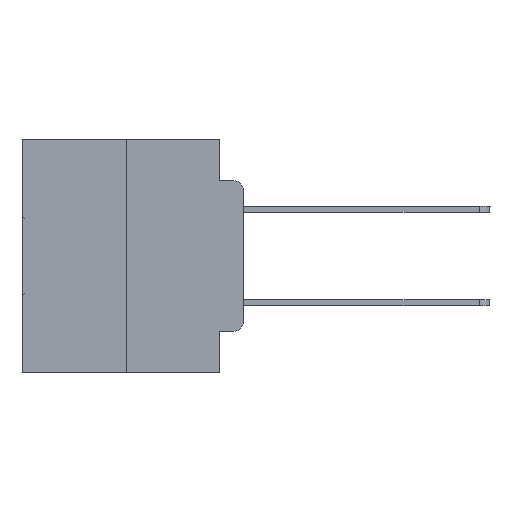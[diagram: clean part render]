
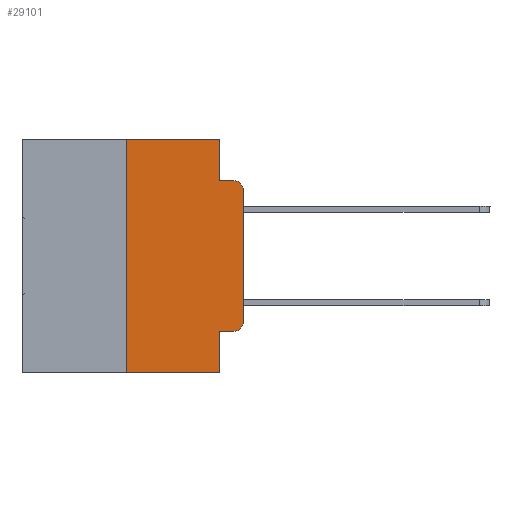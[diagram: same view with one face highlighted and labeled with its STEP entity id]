
A CAD part, left-side view. The second image highlights one B-rep face of the part: STEP entity #29101.
In plain terms, the highlighted planar face has unit normal (-1, 0, 0).
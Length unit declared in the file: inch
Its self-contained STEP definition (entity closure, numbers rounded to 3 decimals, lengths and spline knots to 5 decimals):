
#523 = ORIENTED_EDGE ( 'NONE', *, *, #27543, .T. ) ;
#621 = VERTEX_POINT ( 'NONE', #14830 ) ;
#1143 = CARTESIAN_POINT ( 'NONE',  ( 0., 0.473, 0. ) ) ;
#1203 = VERTEX_POINT ( 'NONE', #7807 ) ;
#1286 = EDGE_LOOP ( 'NONE', ( #523, #7363, #1351, #14677, #22027, #17001, #29893, #12021, #25044, #13533 ) ) ;
#1342 = VERTEX_POINT ( 'NONE', #10955 ) ;
#1351 = ORIENTED_EDGE ( 'NONE', *, *, #3787, .F. ) ;
#1539 = EDGE_CURVE ( 'NONE', #4586, #14637, #24860, .T. ) ;
#1832 = VERTEX_POINT ( 'NONE', #7961 ) ;
#2256 = VECTOR ( 'NONE', #30206, 39.37008 ) ;
#2321 = LINE ( 'NONE', #16980, #14815 ) ;
#2412 = CIRCLE ( 'NONE', #7745, 0.02 ) ;
#2580 = VERTEX_POINT ( 'NONE', #20809 ) ;
#3767 = CARTESIAN_POINT ( 'NONE',  ( 0., 0.051, 0. ) ) ;
#3774 = DIRECTION ( 'NONE',  ( 0., -1., 0. ) ) ;
#3787 = EDGE_CURVE ( 'NONE', #8110, #12003, #15507, .T. ) ;
#3994 = DIRECTION ( 'NONE',  ( 0., -1., 0. ) ) ;
#4586 = VERTEX_POINT ( 'NONE', #30674 ) ;
#6032 = CARTESIAN_POINT ( 'NONE',  ( 0., 0.051, -0.5 ) ) ;
#6189 = LINE ( 'NONE', #25192, #30608 ) ;
#7363 = ORIENTED_EDGE ( 'NONE', *, *, #24331, .T. ) ;
#7745 = AXIS2_PLACEMENT_3D ( 'NONE', #24017, #9310, #26421 ) ;
#7807 = CARTESIAN_POINT ( 'NONE',  ( 0., 0., -0.3915 ) ) ;
#7961 = CARTESIAN_POINT ( 'NONE',  ( 0., 0.25, 0. ) ) ;
#8110 = VERTEX_POINT ( 'NONE', #28149 ) ;
#8748 = VECTOR ( 'NONE', #28116, 39.37008 ) ;
#8820 = DIRECTION ( 'NONE',  ( 1., 0., 0. ) ) ;
#9310 = DIRECTION ( 'NONE',  ( -1., 0., 0. ) ) ;
#9916 = CARTESIAN_POINT ( 'NONE',  ( 0., 0.02, -0.1085 ) ) ;
#10564 = AXIS2_PLACEMENT_3D ( 'NONE', #20979, #8820, #25940 ) ;
#10860 = CARTESIAN_POINT ( 'NONE',  ( 0., 0.051, -0.0885 ) ) ;
#10955 = CARTESIAN_POINT ( 'NONE',  ( 0., 0., -0.1085 ) ) ;
#11109 = EDGE_CURVE ( 'NONE', #4586, #1832, #2321, .T. ) ;
#11284 = VERTEX_POINT ( 'NONE', #19986 ) ;
#12003 = VERTEX_POINT ( 'NONE', #17802 ) ;
#12021 = ORIENTED_EDGE ( 'NONE', *, *, #31860, .F. ) ;
#12216 = CARTESIAN_POINT ( 'NONE',  ( 0., 0.051, -0.4115 ) ) ;
#12369 = DIRECTION ( 'NONE',  ( 0., 0., -1. ) ) ;
#12460 = LINE ( 'NONE', #3767, #25475 ) ;
#13533 = ORIENTED_EDGE ( 'NONE', *, *, #26039, .T. ) ;
#14637 = VERTEX_POINT ( 'NONE', #6032 ) ;
#14677 = ORIENTED_EDGE ( 'NONE', *, *, #25852, .F. ) ;
#14815 = VECTOR ( 'NONE', #19455, 39.37008 ) ;
#14830 = CARTESIAN_POINT ( 'NONE',  ( 0., 0.051, -0.4115 ) ) ;
#15507 = LINE ( 'NONE', #10860, #2256 ) ;
#15982 = LINE ( 'NONE', #12216, #22559 ) ;
#16980 = CARTESIAN_POINT ( 'NONE',  ( 0., 0.25, 0. ) ) ;
#17001 = ORIENTED_EDGE ( 'NONE', *, *, #11109, .F. ) ;
#17802 = CARTESIAN_POINT ( 'NONE',  ( 0., 0.02, -0.0885 ) ) ;
#18014 = AXIS2_PLACEMENT_3D ( 'NONE', #9916, #27007, #12369 ) ;
#18028 = LINE ( 'NONE', #1143, #30133 ) ;
#18337 = VECTOR ( 'NONE', #3994, 39.37008 ) ;
#18910 = EDGE_CURVE ( 'NONE', #621, #2580, #15982, .T. ) ;
#19455 = DIRECTION ( 'NONE',  ( 0., 0., 1. ) ) ;
#19986 = CARTESIAN_POINT ( 'NONE',  ( 0., 0.051, 0. ) ) ;
#20809 = CARTESIAN_POINT ( 'NONE',  ( 0., 0.02, -0.4115 ) ) ;
#20979 = CARTESIAN_POINT ( 'NONE',  ( 0., 0.473, 0. ) ) ;
#21074 = DIRECTION ( 'NONE',  ( 0., 0., -1. ) ) ;
#21130 = CIRCLE ( 'NONE', #18014, 0.02 ) ;
#22027 = ORIENTED_EDGE ( 'NONE', *, *, #29093, .F. ) ;
#22559 = VECTOR ( 'NONE', #26852, 39.37008 ) ;
#23545 = PLANE ( 'NONE',  #10564 ) ;
#23786 = FACE_OUTER_BOUND ( 'NONE', #1286, .T. ) ;
#24017 = CARTESIAN_POINT ( 'NONE',  ( 0., 0.02, -0.3915 ) ) ;
#24331 = EDGE_CURVE ( 'NONE', #1342, #12003, #21130, .T. ) ;
#24860 = LINE ( 'NONE', #27732, #18337 ) ;
#25044 = ORIENTED_EDGE ( 'NONE', *, *, #18910, .T. ) ;
#25192 = CARTESIAN_POINT ( 'NONE',  ( 0., 0., 0. ) ) ;
#25475 = VECTOR ( 'NONE', #21074, 39.37008 ) ;
#25693 = CARTESIAN_POINT ( 'NONE',  ( 0., 0.051, 0. ) ) ;
#25852 = EDGE_CURVE ( 'NONE', #11284, #8110, #27516, .T. ) ;
#25940 = DIRECTION ( 'NONE',  ( 0., 0., -1. ) ) ;
#26039 = EDGE_CURVE ( 'NONE', #2580, #1203, #2412, .T. ) ;
#26421 = DIRECTION ( 'NONE',  ( 0., 0., -1. ) ) ;
#26852 = DIRECTION ( 'NONE',  ( 0., -1., 0. ) ) ;
#27007 = DIRECTION ( 'NONE',  ( -1., 0., 0. ) ) ;
#27516 = LINE ( 'NONE', #25693, #8748 ) ;
#27543 = EDGE_CURVE ( 'NONE', #1203, #1342, #6189, .T. ) ;
#27611 = DIRECTION ( 'NONE',  ( 0., 0., 1. ) ) ;
#27732 = CARTESIAN_POINT ( 'NONE',  ( 0., 0.473, -0.5 ) ) ;
#28116 = DIRECTION ( 'NONE',  ( 0., 0., -1. ) ) ;
#28149 = CARTESIAN_POINT ( 'NONE',  ( 0., 0.051, -0.0885 ) ) ;
#29093 = EDGE_CURVE ( 'NONE', #1832, #11284, #18028, .T. ) ;
#29101 = ADVANCED_FACE ( 'NONE', ( #23786 ), #23545, .F. ) ;
#29893 = ORIENTED_EDGE ( 'NONE', *, *, #1539, .T. ) ;
#30133 = VECTOR ( 'NONE', #3774, 39.37008 ) ;
#30206 = DIRECTION ( 'NONE',  ( 0., -1., 0. ) ) ;
#30608 = VECTOR ( 'NONE', #27611, 39.37008 ) ;
#30674 = CARTESIAN_POINT ( 'NONE',  ( 0., 0.25, -0.5 ) ) ;
#31860 = EDGE_CURVE ( 'NONE', #621, #14637, #12460, .T. ) ;
